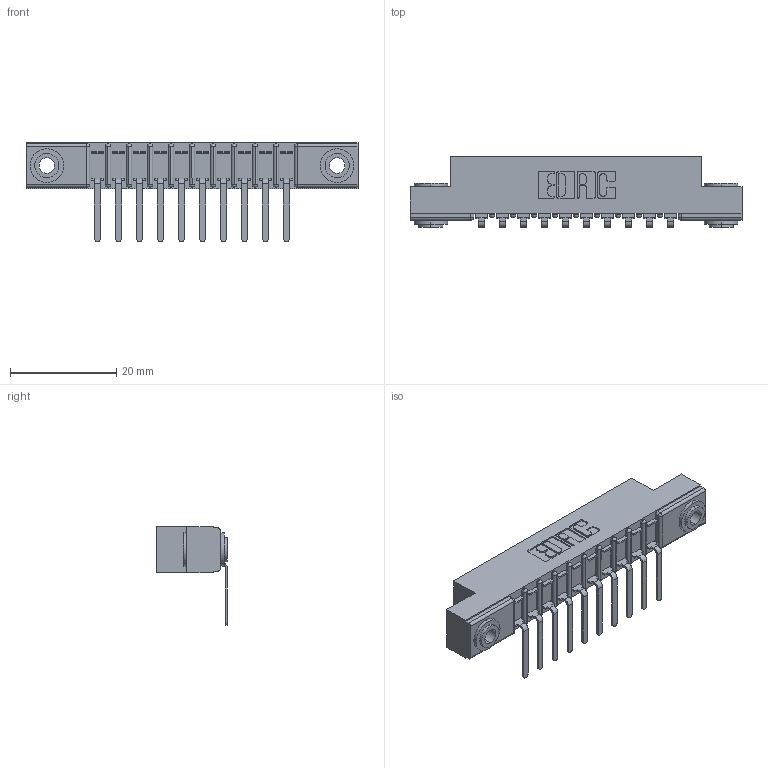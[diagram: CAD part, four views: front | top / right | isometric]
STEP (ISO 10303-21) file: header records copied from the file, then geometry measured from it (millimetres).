
FILE_DESCRIPTION (( 'STEP AP203' ), '1' );
FILE_NAME ('307-010-457-103.STEP', '2020-09-25T08:35:14', ( '' ), ( '' ), 'SwSTEP 2.0', 'SolidWorks 2020', '' );
FILE_SCHEMA (( 'CONFIG_CONTROL_DESIGN' ));
Length unit declared in the file: inch
Products named in the file (4): 307 Part_.156 Dia Mounting Holes; 307-010-457-103; 345-250-002_345-250-002-102; 307-290-002_557
Assembly tree (13 placements, depth 2):
  307-010-457-103
    307 Part_.156 Dia Mounting Holes
    307-290-002_557  x10
    345-250-002_345-250-002-102  x2
Bounding box: 62.64 x 13.36 x 18.67 mm (x, y, z)
Volume: 4157.1 mm3; surface area: 7302.7 mm2
Topology: 13 solids, 13 shells, 961 faces, 2875 edges, 1882 vertices
Faces by surface type: plane 564, cylinder 367, sphere 22, cone 8
Entity records: 14437 total; most frequent: CARTESIAN_POINT 2409, ORIENTED_EDGE 2390, DIRECTION 2371, EDGE_CURVE 1195, LINE 891, VECTOR 891, VERTEX_POINT 778, AXIS2_PLACEMENT_3D 740
